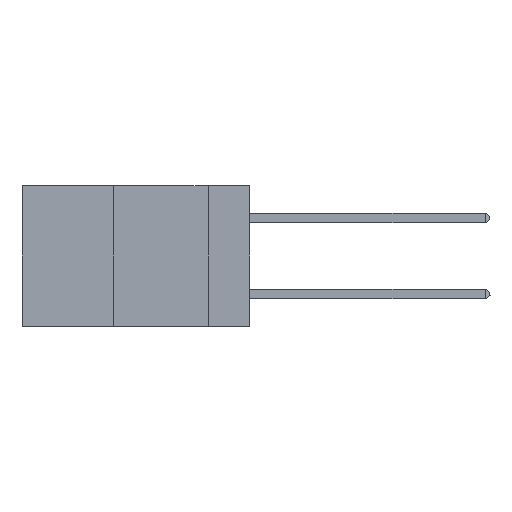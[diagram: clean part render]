
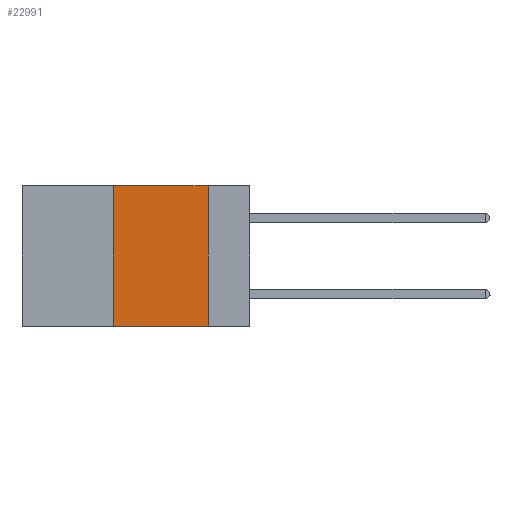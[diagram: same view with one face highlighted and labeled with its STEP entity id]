
A CAD part, left-side view. The second image highlights one B-rep face of the part: STEP entity #22991.
In plain terms, the highlighted planar face has unit normal (-1, 0, 0).
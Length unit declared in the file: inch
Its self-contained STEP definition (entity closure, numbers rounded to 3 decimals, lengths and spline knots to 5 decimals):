
#1049 = LINE ( 'NONE', #8329, #13490 ) ;
#3286 = LINE ( 'NONE', #16740, #7424 ) ;
#3431 = VERTEX_POINT ( 'NONE', #21882 ) ;
#3483 = EDGE_CURVE ( 'NONE', #3431, #11371, #5877, .T. ) ;
#4717 = DIRECTION ( 'NONE',  ( 0., 0., -1. ) ) ;
#5061 = ORIENTED_EDGE ( 'NONE', *, *, #3483, .F. ) ;
#5877 = LINE ( 'NONE', #9694, #8734 ) ;
#6080 = VECTOR ( 'NONE', #4717, 39.37008 ) ;
#6344 = PLANE ( 'NONE',  #15411 ) ;
#6610 = EDGE_CURVE ( 'NONE', #20615, #21259, #7374, .T. ) ;
#7374 = LINE ( 'NONE', #25145, #6080 ) ;
#7424 = VECTOR ( 'NONE', #24803, 39.37008 ) ;
#7858 = ORIENTED_EDGE ( 'NONE', *, *, #6610, .F. ) ;
#8041 = CARTESIAN_POINT ( 'NONE',  ( 0., 0.36, 0. ) ) ;
#8329 = CARTESIAN_POINT ( 'NONE',  ( 0., 0.6, -0.37 ) ) ;
#8734 = VECTOR ( 'NONE', #26122, 39.37008 ) ;
#9694 = CARTESIAN_POINT ( 'NONE',  ( 0., 0.36, 0. ) ) ;
#10700 = CARTESIAN_POINT ( 'NONE',  ( 0., 0.6, 0. ) ) ;
#10789 = DIRECTION ( 'NONE',  ( 1., 0., 0. ) ) ;
#11371 = VERTEX_POINT ( 'NONE', #8041 ) ;
#11427 = ORIENTED_EDGE ( 'NONE', *, *, #11483, .T. ) ;
#11483 = EDGE_CURVE ( 'NONE', #3431, #21259, #1049, .T. ) ;
#12182 = EDGE_CURVE ( 'NONE', #11371, #20615, #3286, .T. ) ;
#12473 = ORIENTED_EDGE ( 'NONE', *, *, #12182, .F. ) ;
#12669 = FACE_OUTER_BOUND ( 'NONE', #25459, .T. ) ;
#13490 = VECTOR ( 'NONE', #18728, 39.37008 ) ;
#15411 = AXIS2_PLACEMENT_3D ( 'NONE', #10700, #10789, #20920 ) ;
#16740 = CARTESIAN_POINT ( 'NONE',  ( 0., 0.6, 0. ) ) ;
#18728 = DIRECTION ( 'NONE',  ( 0., -1., 0. ) ) ;
#20615 = VERTEX_POINT ( 'NONE', #21106 ) ;
#20920 = DIRECTION ( 'NONE',  ( 0., 0., -1. ) ) ;
#21106 = CARTESIAN_POINT ( 'NONE',  ( 0., 0.11, 0. ) ) ;
#21259 = VERTEX_POINT ( 'NONE', #23585 ) ;
#21882 = CARTESIAN_POINT ( 'NONE',  ( 0., 0.36, -0.37 ) ) ;
#22991 = ADVANCED_FACE ( 'NONE', ( #12669 ), #6344, .F. ) ;
#23585 = CARTESIAN_POINT ( 'NONE',  ( 0., 0.11, -0.37 ) ) ;
#24803 = DIRECTION ( 'NONE',  ( 0., -1., 0. ) ) ;
#25145 = CARTESIAN_POINT ( 'NONE',  ( 0., 0.11, 0. ) ) ;
#25459 = EDGE_LOOP ( 'NONE', ( #7858, #12473, #5061, #11427 ) ) ;
#26122 = DIRECTION ( 'NONE',  ( 0., 0., 1. ) ) ;
